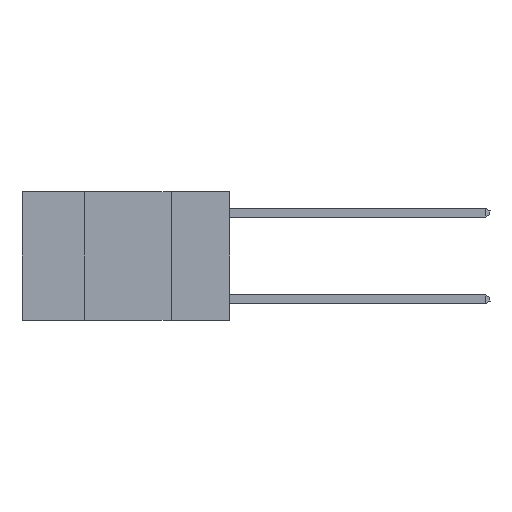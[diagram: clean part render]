
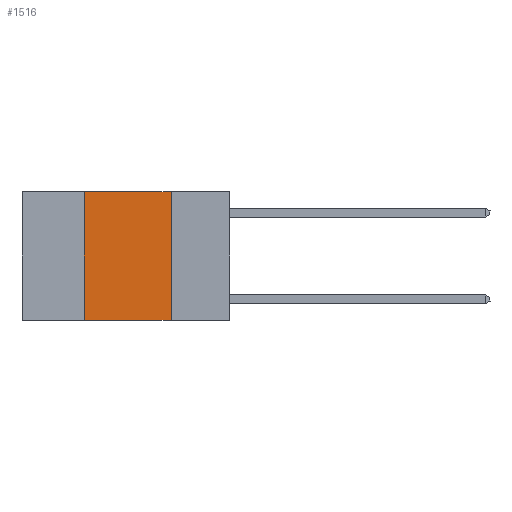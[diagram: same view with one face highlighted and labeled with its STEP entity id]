
A CAD part, left-side view. The second image highlights one B-rep face of the part: STEP entity #1516.
In plain terms, the highlighted planar face has unit normal (-1, 0, 0).
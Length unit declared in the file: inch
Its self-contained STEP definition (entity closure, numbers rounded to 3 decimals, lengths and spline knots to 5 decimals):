
#92 = ORIENTED_EDGE ( 'NONE', *, *, #2882, .F. ) ;
#108 = CARTESIAN_POINT ( 'NONE',  ( 0., 0.6, 0. ) ) ;
#126 = VECTOR ( 'NONE', #6143, 39.37008 ) ;
#203 = ORIENTED_EDGE ( 'NONE', *, *, #11395, .F. ) ;
#447 = CARTESIAN_POINT ( 'NONE',  ( 0., 0.42, 0. ) ) ;
#503 = LINE ( 'NONE', #108, #2440 ) ;
#1267 = DIRECTION ( 'NONE',  ( 0., 0., 1. ) ) ;
#1344 = DIRECTION ( 'NONE',  ( 1., 0., 0. ) ) ;
#1516 = ADVANCED_FACE ( 'NONE', ( #12067 ), #4162, .F. ) ;
#1975 = DIRECTION ( 'NONE',  ( 0., -1., 0. ) ) ;
#2016 = VERTEX_POINT ( 'NONE', #6741 ) ;
#2083 = VECTOR ( 'NONE', #10876, 39.37008 ) ;
#2440 = VECTOR ( 'NONE', #1975, 39.37008 ) ;
#2882 = EDGE_CURVE ( 'NONE', #2016, #3437, #4867, .T. ) ;
#3437 = VERTEX_POINT ( 'NONE', #11657 ) ;
#3821 = AXIS2_PLACEMENT_3D ( 'NONE', #11661, #1344, #7939 ) ;
#4162 = PLANE ( 'NONE',  #3821 ) ;
#4590 = LINE ( 'NONE', #7146, #2083 ) ;
#4867 = LINE ( 'NONE', #11788, #126 ) ;
#5200 = EDGE_CURVE ( 'NONE', #10420, #3437, #4590, .T. ) ;
#6143 = DIRECTION ( 'NONE',  ( 0., 0., -1. ) ) ;
#6360 = LINE ( 'NONE', #11586, #11337 ) ;
#6741 = CARTESIAN_POINT ( 'NONE',  ( 0., 0.17, 0. ) ) ;
#7146 = CARTESIAN_POINT ( 'NONE',  ( 0., 0.6, -0.37 ) ) ;
#7939 = DIRECTION ( 'NONE',  ( 0., 0., -1. ) ) ;
#8504 = EDGE_CURVE ( 'NONE', #10153, #2016, #503, .T. ) ;
#8724 = EDGE_LOOP ( 'NONE', ( #92, #10787, #203, #8821 ) ) ;
#8821 = ORIENTED_EDGE ( 'NONE', *, *, #5200, .T. ) ;
#10153 = VERTEX_POINT ( 'NONE', #447 ) ;
#10420 = VERTEX_POINT ( 'NONE', #12121 ) ;
#10787 = ORIENTED_EDGE ( 'NONE', *, *, #8504, .F. ) ;
#10876 = DIRECTION ( 'NONE',  ( 0., -1., 0. ) ) ;
#11337 = VECTOR ( 'NONE', #1267, 39.37008 ) ;
#11395 = EDGE_CURVE ( 'NONE', #10420, #10153, #6360, .T. ) ;
#11586 = CARTESIAN_POINT ( 'NONE',  ( 0., 0.42, 0. ) ) ;
#11657 = CARTESIAN_POINT ( 'NONE',  ( 0., 0.17, -0.37 ) ) ;
#11661 = CARTESIAN_POINT ( 'NONE',  ( 0., 0.6, 0. ) ) ;
#11788 = CARTESIAN_POINT ( 'NONE',  ( 0., 0.17, 0. ) ) ;
#12067 = FACE_OUTER_BOUND ( 'NONE', #8724, .T. ) ;
#12121 = CARTESIAN_POINT ( 'NONE',  ( 0., 0.42, -0.37 ) ) ;
